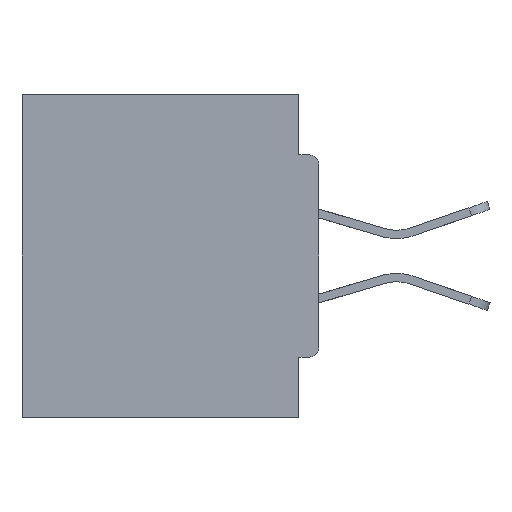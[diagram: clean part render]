
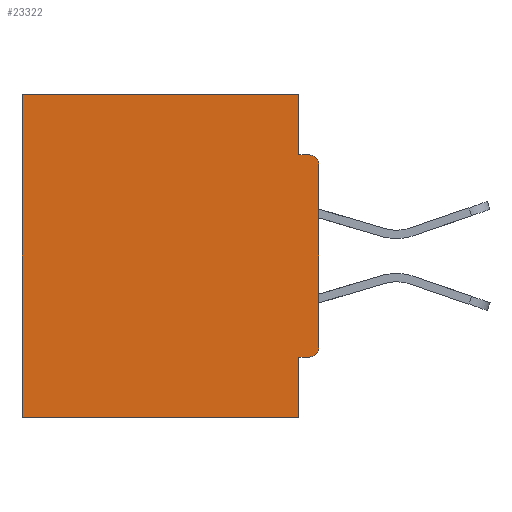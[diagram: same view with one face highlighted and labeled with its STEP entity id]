
A CAD part, left-side view. The second image highlights one B-rep face of the part: STEP entity #23322.
In plain terms, the highlighted planar face has unit normal (-1, 0, 0).
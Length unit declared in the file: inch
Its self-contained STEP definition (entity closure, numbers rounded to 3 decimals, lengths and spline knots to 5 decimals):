
#566 = DIRECTION ( 'NONE',  ( 0., 0., -1. ) ) ;
#969 = VECTOR ( 'NONE', #28732, 39.37008 ) ;
#1124 = ORIENTED_EDGE ( 'NONE', *, *, #20946, .T. ) ;
#1821 = CARTESIAN_POINT ( 'NONE',  ( 0.298, 0.46, 0. ) ) ;
#1964 = AXIS2_PLACEMENT_3D ( 'NONE', #15457, #26117, #25758 ) ;
#2594 = LINE ( 'NONE', #6904, #17918 ) ;
#2630 = CARTESIAN_POINT ( 'NONE',  ( 0.298, 0.015, -0.0935 ) ) ;
#3317 = CARTESIAN_POINT ( 'NONE',  ( 0.298, 0.46, 0. ) ) ;
#3814 = VECTOR ( 'NONE', #30516, 39.37008 ) ;
#4351 = CARTESIAN_POINT ( 'NONE',  ( 0.298, 0., 0. ) ) ;
#4406 = VERTEX_POINT ( 'NONE', #2630 ) ;
#5271 = DIRECTION ( 'NONE',  ( 0., 0., -1. ) ) ;
#5291 = VERTEX_POINT ( 'NONE', #18161 ) ;
#5878 = VERTEX_POINT ( 'NONE', #28395 ) ;
#5915 = ORIENTED_EDGE ( 'NONE', *, *, #21201, .F. ) ;
#6904 = CARTESIAN_POINT ( 'NONE',  ( 0.298, 0., 0. ) ) ;
#7191 = LINE ( 'NONE', #9762, #15085 ) ;
#7998 = ORIENTED_EDGE ( 'NONE', *, *, #27008, .F. ) ;
#8037 = DIRECTION ( 'NONE',  ( 0., 0., -1. ) ) ;
#9644 = LINE ( 'NONE', #21250, #969 ) ;
#9762 = CARTESIAN_POINT ( 'NONE',  ( 0.298, 0., -0.0935 ) ) ;
#9803 = EDGE_CURVE ( 'NONE', #29321, #29696, #2594, .T. ) ;
#11238 = ORIENTED_EDGE ( 'NONE', *, *, #30745, .T. ) ;
#12110 = CARTESIAN_POINT ( 'NONE',  ( 0.298, 0., -0.4065 ) ) ;
#12217 = VECTOR ( 'NONE', #14568, 39.37008 ) ;
#12864 = CARTESIAN_POINT ( 'NONE',  ( 0.298, 0.031, -0.5 ) ) ;
#12886 = ORIENTED_EDGE ( 'NONE', *, *, #26307, .F. ) ;
#12962 = EDGE_CURVE ( 'NONE', #19461, #16367, #29344, .T. ) ;
#13889 = LINE ( 'NONE', #22336, #12217 ) ;
#14568 = DIRECTION ( 'NONE',  ( 0., 0., -1. ) ) ;
#14578 = DIRECTION ( 'NONE',  ( 0., 1., 0. ) ) ;
#15085 = VECTOR ( 'NONE', #33755, 39.37008 ) ;
#15251 = CIRCLE ( 'NONE', #17983, 0.015 ) ;
#15358 = CARTESIAN_POINT ( 'NONE',  ( 0.298, 0., -0.3915 ) ) ;
#15457 = CARTESIAN_POINT ( 'NONE',  ( 0.298, 0.015, -0.1085 ) ) ;
#16351 = CIRCLE ( 'NONE', #1964, 0.015 ) ;
#16367 = VERTEX_POINT ( 'NONE', #32441 ) ;
#16947 = LINE ( 'NONE', #3317, #25188 ) ;
#17443 = DIRECTION ( 'NONE',  ( 0., 1., 0. ) ) ;
#17756 = ORIENTED_EDGE ( 'NONE', *, *, #33660, .T. ) ;
#17918 = VECTOR ( 'NONE', #8037, 39.37008 ) ;
#17983 = AXIS2_PLACEMENT_3D ( 'NONE', #29011, #21181, #5271 ) ;
#18137 = DIRECTION ( 'NONE',  ( 0., 0., -1. ) ) ;
#18161 = CARTESIAN_POINT ( 'NONE',  ( 0.298, 0.015, -0.4065 ) ) ;
#18311 = VERTEX_POINT ( 'NONE', #29612 ) ;
#19461 = VERTEX_POINT ( 'NONE', #12864 ) ;
#19622 = VERTEX_POINT ( 'NONE', #26860 ) ;
#20682 = CARTESIAN_POINT ( 'NONE',  ( 0.298, 0., 0. ) ) ;
#20946 = EDGE_CURVE ( 'NONE', #5291, #29696, #15251, .T. ) ;
#21033 = PLANE ( 'NONE',  #25768 ) ;
#21181 = DIRECTION ( 'NONE',  ( -1., 0., 0. ) ) ;
#21201 = EDGE_CURVE ( 'NONE', #5291, #19622, #30559, .T. ) ;
#21250 = CARTESIAN_POINT ( 'NONE',  ( 0.298, 0.031, -0.5 ) ) ;
#22336 = CARTESIAN_POINT ( 'NONE',  ( 0.298, 0.031, -0.5 ) ) ;
#22649 = ORIENTED_EDGE ( 'NONE', *, *, #28111, .T. ) ;
#23322 = ADVANCED_FACE ( 'NONE', ( #25893 ), #21033, .F. ) ;
#24995 = CARTESIAN_POINT ( 'NONE',  ( 0.298, 0., -0.5 ) ) ;
#25188 = VECTOR ( 'NONE', #566, 39.37008 ) ;
#25758 = DIRECTION ( 'NONE',  ( 0., 0., -1. ) ) ;
#25768 = AXIS2_PLACEMENT_3D ( 'NONE', #20682, #26338, #18137 ) ;
#25780 = LINE ( 'NONE', #4351, #3814 ) ;
#25893 = FACE_OUTER_BOUND ( 'NONE', #27390, .T. ) ;
#26117 = DIRECTION ( 'NONE',  ( -1., 0., 0. ) ) ;
#26176 = ORIENTED_EDGE ( 'NONE', *, *, #27362, .F. ) ;
#26307 = EDGE_CURVE ( 'NONE', #19622, #19461, #13889, .T. ) ;
#26338 = DIRECTION ( 'NONE',  ( 1., 0., 0. ) ) ;
#26860 = CARTESIAN_POINT ( 'NONE',  ( 0.298, 0.031, -0.4065 ) ) ;
#27008 = EDGE_CURVE ( 'NONE', #18311, #4406, #7191, .T. ) ;
#27087 = CARTESIAN_POINT ( 'NONE',  ( 0.298, 0., -0.1085 ) ) ;
#27362 = EDGE_CURVE ( 'NONE', #5878, #18311, #9644, .T. ) ;
#27390 = EDGE_LOOP ( 'NONE', ( #11238, #7998, #26176, #22649, #17756, #33515, #12886, #5915, #1124, #32343 ) ) ;
#28111 = EDGE_CURVE ( 'NONE', #5878, #33851, #25780, .T. ) ;
#28395 = CARTESIAN_POINT ( 'NONE',  ( 0.298, 0.031, 0. ) ) ;
#28732 = DIRECTION ( 'NONE',  ( 0., 0., -1. ) ) ;
#29011 = CARTESIAN_POINT ( 'NONE',  ( 0.298, 0.015, -0.3915 ) ) ;
#29321 = VERTEX_POINT ( 'NONE', #27087 ) ;
#29344 = LINE ( 'NONE', #24995, #32243 ) ;
#29612 = CARTESIAN_POINT ( 'NONE',  ( 0.298, 0.031, -0.0935 ) ) ;
#29696 = VERTEX_POINT ( 'NONE', #15358 ) ;
#30516 = DIRECTION ( 'NONE',  ( 0., 1., 0. ) ) ;
#30559 = LINE ( 'NONE', #12110, #32633 ) ;
#30745 = EDGE_CURVE ( 'NONE', #29321, #4406, #16351, .T. ) ;
#32243 = VECTOR ( 'NONE', #14578, 39.37008 ) ;
#32343 = ORIENTED_EDGE ( 'NONE', *, *, #9803, .F. ) ;
#32441 = CARTESIAN_POINT ( 'NONE',  ( 0.298, 0.46, -0.5 ) ) ;
#32633 = VECTOR ( 'NONE', #17443, 39.37008 ) ;
#33515 = ORIENTED_EDGE ( 'NONE', *, *, #12962, .F. ) ;
#33660 = EDGE_CURVE ( 'NONE', #33851, #16367, #16947, .T. ) ;
#33755 = DIRECTION ( 'NONE',  ( 0., -1., 0. ) ) ;
#33851 = VERTEX_POINT ( 'NONE', #1821 ) ;
